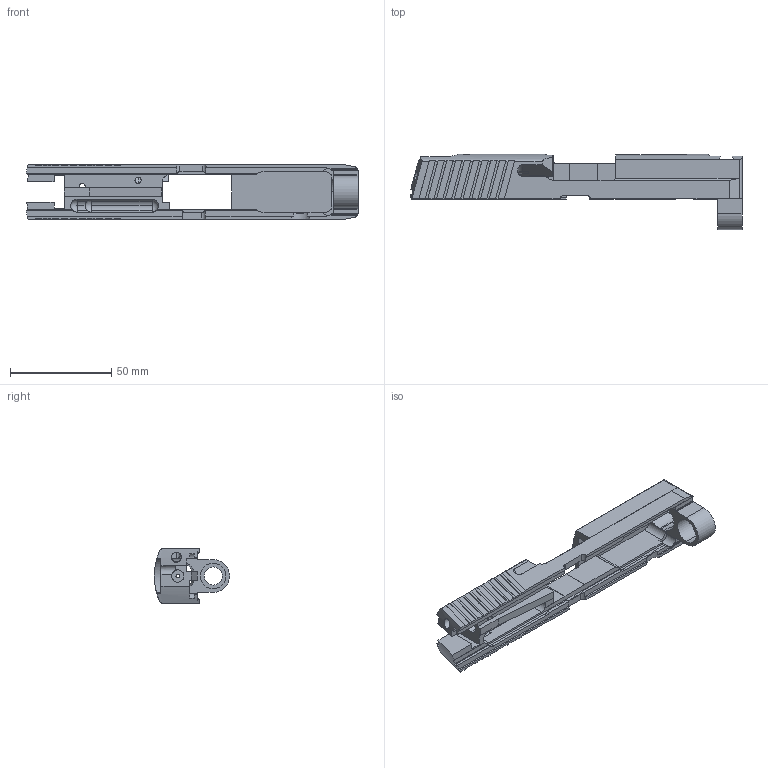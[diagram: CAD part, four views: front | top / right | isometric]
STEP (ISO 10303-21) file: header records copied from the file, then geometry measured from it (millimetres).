
FILE_DESCRIPTION (( 'STEP AP214' ), '1' );
FILE_NAME ('Slide_1.step', '2014-07-30T19:46:56', ( 'WarFairy' ), ( '' ), 'SwSTEP 2.0', 'SolidWorks 2013', '' );
FILE_SCHEMA (( 'AUTOMOTIVE_DESIGN' ));
Length unit declared in the file: millimetre
Products named in the file (1): Slide_1
Bounding box: 164.01 x 37.16 x 26.78 mm (x, y, z)
Volume: 36975.4 mm3; surface area: 24600.6 mm2
Topology: 1 solids, 1 shells, 702 faces, 2014 edges, 1335 vertices
Faces by surface type: plane 427, bspline 180, cylinder 90, torus 3, cone 2
Entity records: 24546 total; most frequent: CARTESIAN_POINT 7428, ORIENTED_EDGE 4024, DIRECTION 2756, EDGE_CURVE 2012, VECTOR 1356, LINE 1356, VERTEX_POINT 1335, EDGE_LOOP 743
